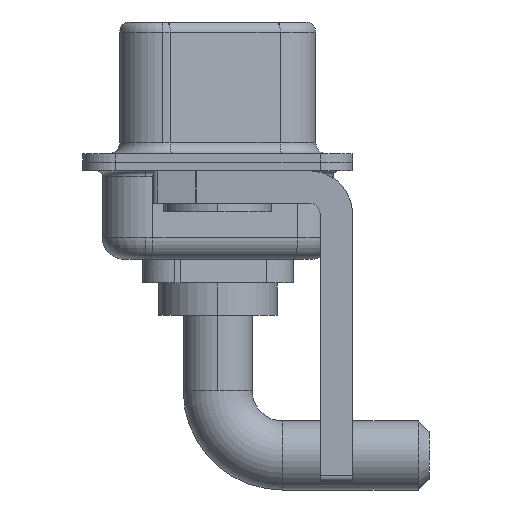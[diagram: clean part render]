
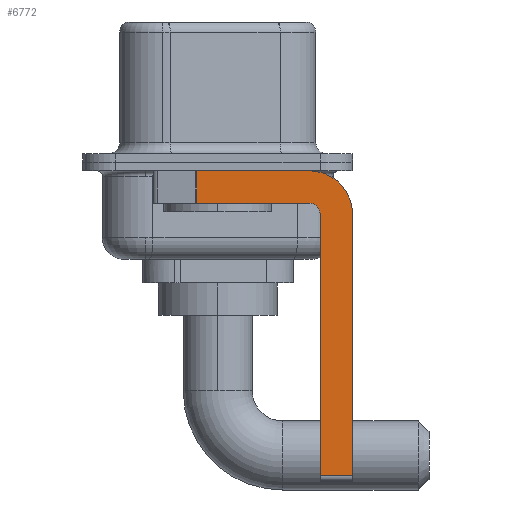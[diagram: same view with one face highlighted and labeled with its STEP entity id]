
A CAD part, left-side view. The second image highlights one B-rep face of the part: STEP entity #6772.
In plain terms, the highlighted planar face has unit normal (-1, 0, 0).
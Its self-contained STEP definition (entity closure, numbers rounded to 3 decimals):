
#156 = EDGE_CURVE ( 'NONE', #5629, #14163, #2557, .T. ) ;
#859 = ORIENTED_EDGE ( 'NONE', *, *, #15648, .F. ) ;
#1195 = PLANE ( 'NONE',  #15052 ) ;
#1259 = CARTESIAN_POINT ( 'NONE',  ( -2.9, -4.25, -0.4 ) ) ;
#1356 = DIRECTION ( 'NONE',  ( 0., 0., -1. ) ) ;
#1657 = EDGE_LOOP ( 'NONE', ( #16628, #4654, #4594, #859, #15995, #14706, #14739, #13328 ) ) ;
#2557 = LINE ( 'NONE', #8118, #12954 ) ;
#2686 = LINE ( 'NONE', #8078, #12007 ) ;
#3486 = EDGE_CURVE ( 'NONE', #5397, #14163, #6732, .T. ) ;
#3877 = CIRCLE ( 'NONE', #12074, 0.5 ) ;
#4594 = ORIENTED_EDGE ( 'NONE', *, *, #16572, .F. ) ;
#4654 = ORIENTED_EDGE ( 'NONE', *, *, #12674, .T. ) ;
#4919 = EDGE_CURVE ( 'NONE', #7214, #5397, #16593, .T. ) ;
#5184 = VECTOR ( 'NONE', #10223, 1000. ) ;
#5378 = DIRECTION ( 'NONE',  ( 0., -1., 0. ) ) ;
#5397 = VERTEX_POINT ( 'NONE', #11602 ) ;
#5629 = VERTEX_POINT ( 'NONE', #10739 ) ;
#5874 = CARTESIAN_POINT ( 'NONE',  ( -2.9, 3., -0.4 ) ) ;
#5959 = CARTESIAN_POINT ( 'NONE',  ( -2.9, 0.978, -0.4 ) ) ;
#6006 = CARTESIAN_POINT ( 'NONE',  ( -2.9, -4.25, -2.4 ) ) ;
#6223 = CARTESIAN_POINT ( 'NONE',  ( -2.9, 0.978, -1.9 ) ) ;
#6363 = VECTOR ( 'NONE', #16347, 1000. ) ;
#6551 = CARTESIAN_POINT ( 'NONE',  ( -2.9, -4.25, -2.4 ) ) ;
#6732 = LINE ( 'NONE', #6818, #8407 ) ;
#6772 = ADVANCED_FACE ( 'NONE', ( #14319 ), #1195, .F. ) ;
#6805 = VERTEX_POINT ( 'NONE', #6223 ) ;
#6818 = CARTESIAN_POINT ( 'NONE',  ( -2.9, -6.25, -2.4 ) ) ;
#7214 = VERTEX_POINT ( 'NONE', #1259 ) ;
#7346 = CARTESIAN_POINT ( 'NONE',  ( -2.9, -4.25, -1.9 ) ) ;
#7402 = LINE ( 'NONE', #15221, #12373 ) ;
#7508 = DIRECTION ( 'NONE',  ( 0., 0., -1. ) ) ;
#7767 = CARTESIAN_POINT ( 'NONE',  ( -2.9, -4.25, -2.4 ) ) ;
#7903 = DIRECTION ( 'NONE',  ( 0., 0., 1. ) ) ;
#8078 = CARTESIAN_POINT ( 'NONE',  ( -2.9, -4.75, -14.8 ) ) ;
#8118 = CARTESIAN_POINT ( 'NONE',  ( -2.9, -4.25, -14.55 ) ) ;
#8407 = VECTOR ( 'NONE', #1356, 1000. ) ;
#8442 = AXIS2_PLACEMENT_3D ( 'NONE', #6006, #9941, #15111 ) ;
#8698 = CARTESIAN_POINT ( 'NONE',  ( -2.9, 0.978, -1.9 ) ) ;
#9201 = DIRECTION ( 'NONE',  ( 0., 0., 1. ) ) ;
#9941 = DIRECTION ( 'NONE',  ( 1., 0., 0. ) ) ;
#10223 = DIRECTION ( 'NONE',  ( 0., 0., -1. ) ) ;
#10739 = CARTESIAN_POINT ( 'NONE',  ( -2.9, -4.75, -14.55 ) ) ;
#11602 = CARTESIAN_POINT ( 'NONE',  ( -2.9, -6.25, -2.4 ) ) ;
#11768 = DIRECTION ( 'NONE',  ( -1., 0., 0. ) ) ;
#12007 = VECTOR ( 'NONE', #7903, 1000. ) ;
#12074 = AXIS2_PLACEMENT_3D ( 'NONE', #6551, #11768, #9201 ) ;
#12373 = VECTOR ( 'NONE', #12613, 1000. ) ;
#12545 = VERTEX_POINT ( 'NONE', #5959 ) ;
#12613 = DIRECTION ( 'NONE',  ( 0., 1., 0. ) ) ;
#12674 = EDGE_CURVE ( 'NONE', #12545, #6805, #12860, .T. ) ;
#12799 = EDGE_CURVE ( 'NONE', #5629, #14871, #2686, .T. ) ;
#12860 = LINE ( 'NONE', #8698, #5184 ) ;
#12954 = VECTOR ( 'NONE', #5378, 1000. ) ;
#13027 = CARTESIAN_POINT ( 'NONE',  ( -2.9, -6.25, -14.55 ) ) ;
#13328 = ORIENTED_EDGE ( 'NONE', *, *, #4919, .F. ) ;
#13337 = CARTESIAN_POINT ( 'NONE',  ( -2.9, -4.75, -2.4 ) ) ;
#13507 = VERTEX_POINT ( 'NONE', #7346 ) ;
#13864 = LINE ( 'NONE', #5874, #6363 ) ;
#14163 = VERTEX_POINT ( 'NONE', #13027 ) ;
#14319 = FACE_OUTER_BOUND ( 'NONE', #1657, .T. ) ;
#14706 = ORIENTED_EDGE ( 'NONE', *, *, #156, .T. ) ;
#14739 = ORIENTED_EDGE ( 'NONE', *, *, #3486, .F. ) ;
#14871 = VERTEX_POINT ( 'NONE', #13337 ) ;
#15052 = AXIS2_PLACEMENT_3D ( 'NONE', #7767, #15414, #7508 ) ;
#15111 = DIRECTION ( 'NONE',  ( 0., 0., -1. ) ) ;
#15221 = CARTESIAN_POINT ( 'NONE',  ( -2.9, -4.25, -1.9 ) ) ;
#15414 = DIRECTION ( 'NONE',  ( 1., 0., 0. ) ) ;
#15648 = EDGE_CURVE ( 'NONE', #14871, #13507, #3877, .T. ) ;
#15995 = ORIENTED_EDGE ( 'NONE', *, *, #12799, .F. ) ;
#16347 = DIRECTION ( 'NONE',  ( 0., -1., 0. ) ) ;
#16524 = EDGE_CURVE ( 'NONE', #12545, #7214, #13864, .T. ) ;
#16572 = EDGE_CURVE ( 'NONE', #13507, #6805, #7402, .T. ) ;
#16593 = CIRCLE ( 'NONE', #8442, 2. ) ;
#16628 = ORIENTED_EDGE ( 'NONE', *, *, #16524, .F. ) ;
